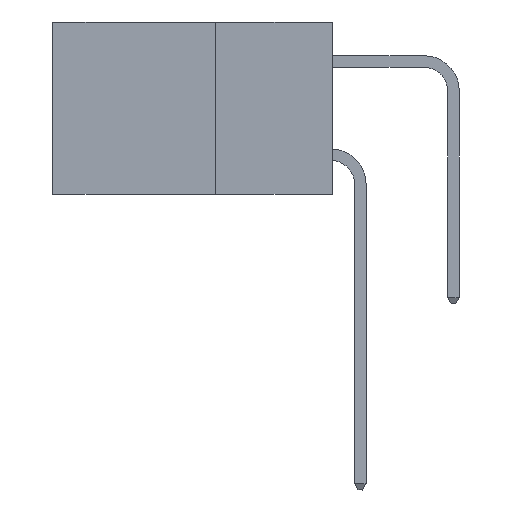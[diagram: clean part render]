
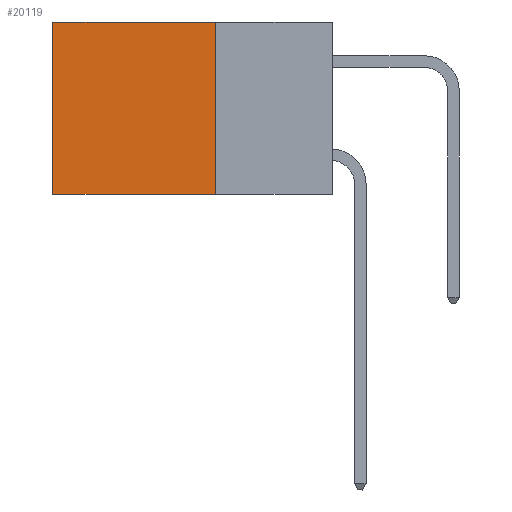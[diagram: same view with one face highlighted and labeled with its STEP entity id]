
A CAD part, left-side view. The second image highlights one B-rep face of the part: STEP entity #20119.
In plain terms, the highlighted planar face has unit normal (-1, 0, 0).
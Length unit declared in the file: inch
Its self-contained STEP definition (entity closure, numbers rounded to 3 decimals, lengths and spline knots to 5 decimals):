
#678 = DIRECTION ( 'NONE',  ( 1., 0., 0. ) ) ;
#1083 = LINE ( 'NONE', #16970, #27111 ) ;
#2314 = VECTOR ( 'NONE', #15288, 39.37008 ) ;
#2333 = DIRECTION ( 'NONE',  ( 0., 0., -1. ) ) ;
#2889 = EDGE_CURVE ( 'NONE', #14522, #23733, #13360, .T. ) ;
#2906 = FACE_OUTER_BOUND ( 'NONE', #18641, .T. ) ;
#4878 = EDGE_CURVE ( 'NONE', #19535, #14522, #1083, .T. ) ;
#6261 = CARTESIAN_POINT ( 'NONE',  ( 0.2615, 0.25, -0.37 ) ) ;
#6953 = CARTESIAN_POINT ( 'NONE',  ( 0.2615, 0.25, 0. ) ) ;
#7088 = CARTESIAN_POINT ( 'NONE',  ( 0.2615, 0.25, -0.37 ) ) ;
#8327 = DIRECTION ( 'NONE',  ( 0., 0., -1. ) ) ;
#8480 = CARTESIAN_POINT ( 'NONE',  ( 0.2615, 0.6, -0.37 ) ) ;
#10062 = CARTESIAN_POINT ( 'NONE',  ( 0.2615, 0.6, -0.37 ) ) ;
#10393 = VERTEX_POINT ( 'NONE', #14909 ) ;
#12746 = ORIENTED_EDGE ( 'NONE', *, *, #2889, .F. ) ;
#13360 = LINE ( 'NONE', #6261, #2314 ) ;
#14522 = VERTEX_POINT ( 'NONE', #21738 ) ;
#14571 = VECTOR ( 'NONE', #8327, 39.37008 ) ;
#14821 = VECTOR ( 'NONE', #20157, 39.37008 ) ;
#14909 = CARTESIAN_POINT ( 'NONE',  ( 0.2615, 0.6, 0. ) ) ;
#15288 = DIRECTION ( 'NONE',  ( 0., 1., 0. ) ) ;
#15317 = EDGE_CURVE ( 'NONE', #10393, #23733, #26436, .T. ) ;
#16970 = CARTESIAN_POINT ( 'NONE',  ( 0.2615, 0.25, -0.37 ) ) ;
#18360 = PLANE ( 'NONE',  #22344 ) ;
#18641 = EDGE_LOOP ( 'NONE', ( #28113, #12746, #23601, #26139 ) ) ;
#19535 = VERTEX_POINT ( 'NONE', #22124 ) ;
#20119 = ADVANCED_FACE ( 'NONE', ( #2906 ), #18360, .F. ) ;
#20157 = DIRECTION ( 'NONE',  ( 0., 1., 0. ) ) ;
#20738 = LINE ( 'NONE', #6953, #14821 ) ;
#21738 = CARTESIAN_POINT ( 'NONE',  ( 0.2615, 0.25, -0.37 ) ) ;
#22124 = CARTESIAN_POINT ( 'NONE',  ( 0.2615, 0.25, 0. ) ) ;
#22292 = EDGE_CURVE ( 'NONE', #19535, #10393, #20738, .T. ) ;
#22344 = AXIS2_PLACEMENT_3D ( 'NONE', #7088, #678, #2333 ) ;
#23601 = ORIENTED_EDGE ( 'NONE', *, *, #4878, .F. ) ;
#23733 = VERTEX_POINT ( 'NONE', #10062 ) ;
#26042 = DIRECTION ( 'NONE',  ( 0., 0., -1. ) ) ;
#26139 = ORIENTED_EDGE ( 'NONE', *, *, #22292, .T. ) ;
#26436 = LINE ( 'NONE', #8480, #14571 ) ;
#27111 = VECTOR ( 'NONE', #26042, 39.37008 ) ;
#28113 = ORIENTED_EDGE ( 'NONE', *, *, #15317, .T. ) ;
